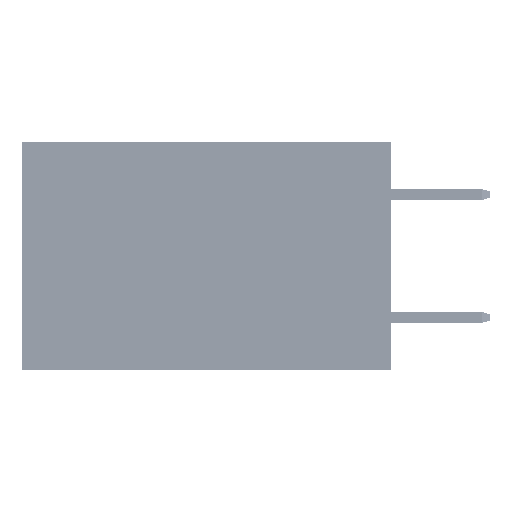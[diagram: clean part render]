
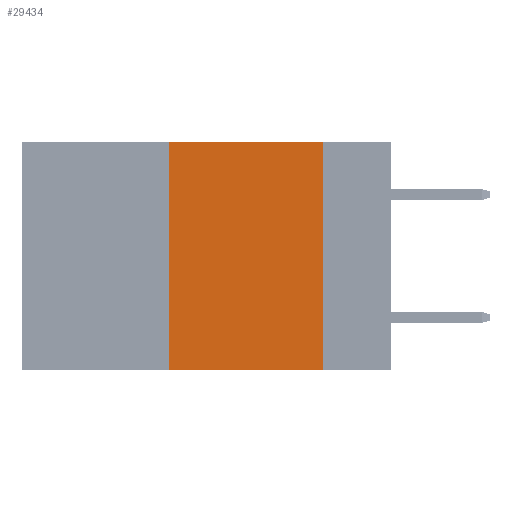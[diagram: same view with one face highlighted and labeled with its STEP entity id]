
A CAD part, left-side view. The second image highlights one B-rep face of the part: STEP entity #29434.
In plain terms, the highlighted planar face has unit normal (-1, 0, 0).
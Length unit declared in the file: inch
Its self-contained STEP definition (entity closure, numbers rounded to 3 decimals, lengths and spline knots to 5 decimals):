
#1 = DIRECTION ( 'NONE',  ( 0., 0., 1. ) ) ;
#289 = VECTOR ( 'NONE', #7128, 39.37008 ) ;
#1429 = DIRECTION ( 'NONE',  ( 0., -1., 0. ) ) ;
#1748 = LINE ( 'NONE', #48746, #8770 ) ;
#2389 = DIRECTION ( 'NONE',  ( 0., 0., -1. ) ) ;
#4000 = FACE_OUTER_BOUND ( 'NONE', #6659, .T. ) ;
#6323 = LINE ( 'NONE', #30336, #19670 ) ;
#6659 = EDGE_LOOP ( 'NONE', ( #7270, #35063, #32530, #11634 ) ) ;
#7128 = DIRECTION ( 'NONE',  ( 0., -1., 0. ) ) ;
#7270 = ORIENTED_EDGE ( 'NONE', *, *, #31413, .F. ) ;
#8770 = VECTOR ( 'NONE', #1, 39.37008 ) ;
#9134 = CARTESIAN_POINT ( 'NONE',  ( 0., 0.6, 0. ) ) ;
#11634 = ORIENTED_EDGE ( 'NONE', *, *, #44830, .T. ) ;
#14577 = CARTESIAN_POINT ( 'NONE',  ( 0., 0.11, 0. ) ) ;
#14763 = CARTESIAN_POINT ( 'NONE',  ( 0., 0.6, -0.37 ) ) ;
#15142 = EDGE_CURVE ( 'NONE', #39381, #48332, #44296, .T. ) ;
#19670 = VECTOR ( 'NONE', #42908, 39.37008 ) ;
#19989 = CARTESIAN_POINT ( 'NONE',  ( 0., 0.11, -0.37 ) ) ;
#20760 = VERTEX_POINT ( 'NONE', #41057 ) ;
#29434 = ADVANCED_FACE ( 'NONE', ( #4000 ), #29657, .F. ) ;
#29657 = PLANE ( 'NONE',  #30702 ) ;
#30336 = CARTESIAN_POINT ( 'NONE',  ( 0., 0.11, 0. ) ) ;
#30702 = AXIS2_PLACEMENT_3D ( 'NONE', #47183, #34777, #2389 ) ;
#31413 = EDGE_CURVE ( 'NONE', #48332, #40856, #6323, .T. ) ;
#32530 = ORIENTED_EDGE ( 'NONE', *, *, #32981, .F. ) ;
#32981 = EDGE_CURVE ( 'NONE', #20760, #39381, #1748, .T. ) ;
#34777 = DIRECTION ( 'NONE',  ( 1., 0., 0. ) ) ;
#34790 = VECTOR ( 'NONE', #1429, 39.37008 ) ;
#35063 = ORIENTED_EDGE ( 'NONE', *, *, #15142, .F. ) ;
#37909 = LINE ( 'NONE', #14763, #289 ) ;
#38381 = CARTESIAN_POINT ( 'NONE',  ( 0., 0.36, 0. ) ) ;
#39381 = VERTEX_POINT ( 'NONE', #38381 ) ;
#40856 = VERTEX_POINT ( 'NONE', #19989 ) ;
#41057 = CARTESIAN_POINT ( 'NONE',  ( 0., 0.36, -0.37 ) ) ;
#42908 = DIRECTION ( 'NONE',  ( 0., 0., -1. ) ) ;
#44296 = LINE ( 'NONE', #9134, #34790 ) ;
#44830 = EDGE_CURVE ( 'NONE', #20760, #40856, #37909, .T. ) ;
#47183 = CARTESIAN_POINT ( 'NONE',  ( 0., 0.6, 0. ) ) ;
#48332 = VERTEX_POINT ( 'NONE', #14577 ) ;
#48746 = CARTESIAN_POINT ( 'NONE',  ( 0., 0.36, 0. ) ) ;
